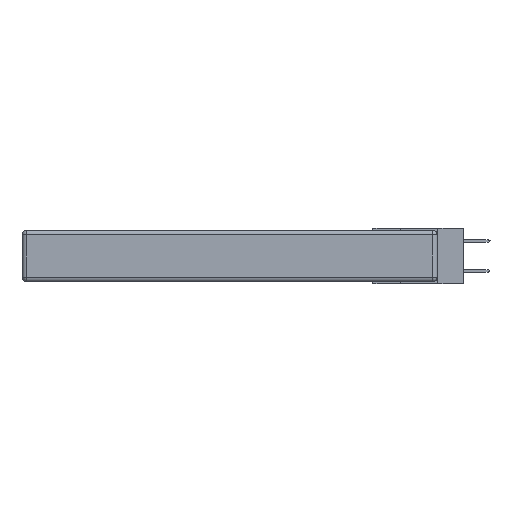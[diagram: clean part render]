
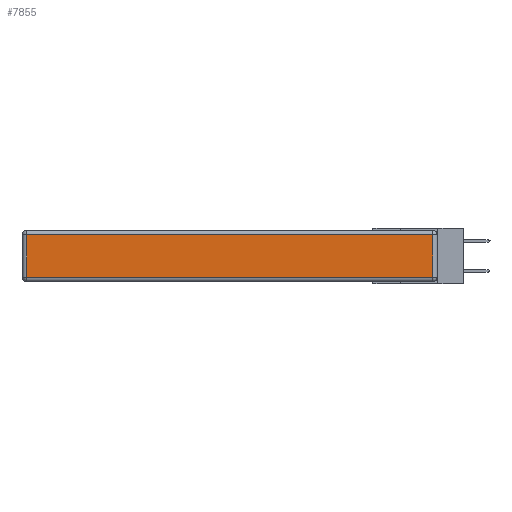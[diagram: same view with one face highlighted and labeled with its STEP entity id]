
A CAD part, left-side view. The second image highlights one B-rep face of the part: STEP entity #7855.
In plain terms, the highlighted planar face has unit normal (-1, 0, 0).
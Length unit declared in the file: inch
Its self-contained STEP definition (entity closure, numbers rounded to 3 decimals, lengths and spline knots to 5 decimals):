
#1112 = CARTESIAN_POINT ( 'NONE',  ( 0., 0.03, -0.313 ) ) ;
#1368 = ORIENTED_EDGE ( 'NONE', *, *, #4995, .T. ) ;
#1671 = LINE ( 'NONE', #8619, #10227 ) ;
#1770 = CARTESIAN_POINT ( 'NONE',  ( 0., 2.72, -0.313 ) ) ;
#1946 = DIRECTION ( 'NONE',  ( 0., -1., 0. ) ) ;
#3688 = CARTESIAN_POINT ( 'NONE',  ( 0., 2.75, -0.03 ) ) ;
#4314 = LINE ( 'NONE', #3688, #11951 ) ;
#4678 = CARTESIAN_POINT ( 'NONE',  ( 0., 0., -0.343 ) ) ;
#4995 = EDGE_CURVE ( 'NONE', #17362, #14197, #16199, .T. ) ;
#6047 = CARTESIAN_POINT ( 'NONE',  ( 0., 0., -0.313 ) ) ;
#6631 = FACE_OUTER_BOUND ( 'NONE', #10562, .T. ) ;
#6762 = DIRECTION ( 'NONE',  ( 0., 0., -1. ) ) ;
#7844 = ORIENTED_EDGE ( 'NONE', *, *, #11671, .T. ) ;
#7855 = ADVANCED_FACE ( 'NONE', ( #6631 ), #13057, .T. ) ;
#8209 = ORIENTED_EDGE ( 'NONE', *, *, #10320, .T. ) ;
#8619 = CARTESIAN_POINT ( 'NONE',  ( 0., 0.03, -0.343 ) ) ;
#9057 = ORIENTED_EDGE ( 'NONE', *, *, #14482, .T. ) ;
#9253 = DIRECTION ( 'NONE',  ( 0., 0., 1. ) ) ;
#9363 = CARTESIAN_POINT ( 'NONE',  ( 0., 2.72, -0.03 ) ) ;
#10227 = VECTOR ( 'NONE', #9253, 39.37008 ) ;
#10320 = EDGE_CURVE ( 'NONE', #14197, #14136, #14457, .T. ) ;
#10562 = EDGE_LOOP ( 'NONE', ( #8209, #7844, #9057, #1368 ) ) ;
#11082 = CARTESIAN_POINT ( 'NONE',  ( 0., 2.72, -0.343 ) ) ;
#11671 = EDGE_CURVE ( 'NONE', #14136, #14750, #1671, .T. ) ;
#11951 = VECTOR ( 'NONE', #12111, 39.37008 ) ;
#12111 = DIRECTION ( 'NONE',  ( 0., 1., 0. ) ) ;
#12495 = VECTOR ( 'NONE', #6762, 39.37008 ) ;
#13057 = PLANE ( 'NONE',  #13232 ) ;
#13232 = AXIS2_PLACEMENT_3D ( 'NONE', #4678, #14474, #17118 ) ;
#13786 = VECTOR ( 'NONE', #1946, 39.37008 ) ;
#14064 = CARTESIAN_POINT ( 'NONE',  ( 0., 0.03, -0.03 ) ) ;
#14136 = VERTEX_POINT ( 'NONE', #1112 ) ;
#14197 = VERTEX_POINT ( 'NONE', #1770 ) ;
#14457 = LINE ( 'NONE', #6047, #13786 ) ;
#14474 = DIRECTION ( 'NONE',  ( -1., 0., 0. ) ) ;
#14482 = EDGE_CURVE ( 'NONE', #14750, #17362, #4314, .T. ) ;
#14750 = VERTEX_POINT ( 'NONE', #14064 ) ;
#16199 = LINE ( 'NONE', #11082, #12495 ) ;
#17118 = DIRECTION ( 'NONE',  ( 0., 0., 1. ) ) ;
#17362 = VERTEX_POINT ( 'NONE', #9363 ) ;
